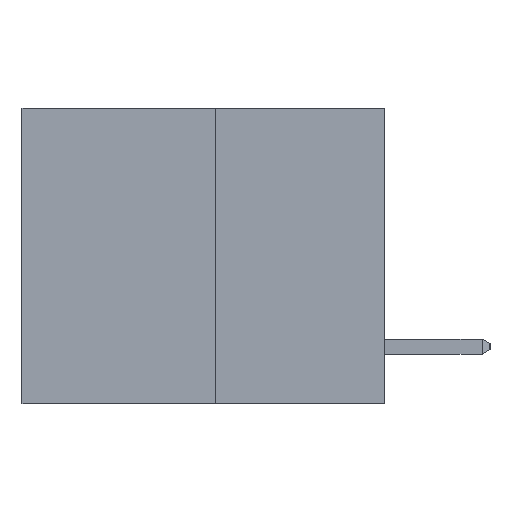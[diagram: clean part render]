
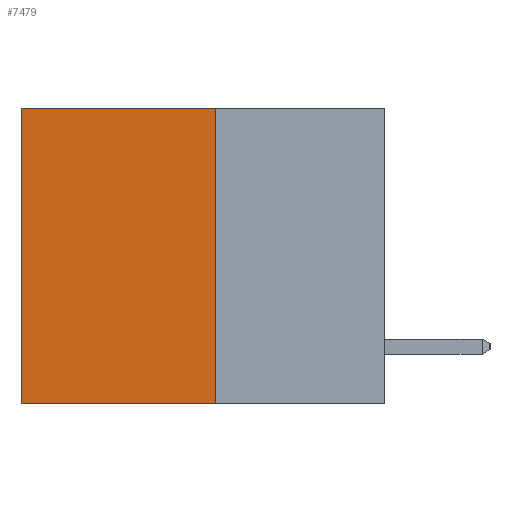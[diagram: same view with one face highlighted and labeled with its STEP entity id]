
A CAD part, left-side view. The second image highlights one B-rep face of the part: STEP entity #7479.
In plain terms, the highlighted planar face has unit normal (-1, 0, 0).
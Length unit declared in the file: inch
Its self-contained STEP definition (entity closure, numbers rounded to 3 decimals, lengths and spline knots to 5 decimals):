
#3 = EDGE_CURVE ( 'NONE', #7090, #13410, #5856, .T. ) ;
#806 = DIRECTION ( 'NONE',  ( 0., 0., -1. ) ) ;
#879 = ORIENTED_EDGE ( 'NONE', *, *, #5650, .T. ) ;
#2530 = CARTESIAN_POINT ( 'NONE',  ( 0.3165, 0.28, 0. ) ) ;
#3694 = LINE ( 'NONE', #10502, #8239 ) ;
#3913 = DIRECTION ( 'NONE',  ( 0., 0., -1. ) ) ;
#5212 = CARTESIAN_POINT ( 'NONE',  ( 0.3165, 0.6, -0.49 ) ) ;
#5503 = LINE ( 'NONE', #7113, #12118 ) ;
#5650 = EDGE_CURVE ( 'NONE', #7469, #7090, #3694, .T. ) ;
#5856 = LINE ( 'NONE', #9964, #11544 ) ;
#5932 = EDGE_LOOP ( 'NONE', ( #9068, #12618, #8755, #879 ) ) ;
#6131 = DIRECTION ( 'NONE',  ( 1., 0., 0. ) ) ;
#7090 = VERTEX_POINT ( 'NONE', #12111 ) ;
#7113 = CARTESIAN_POINT ( 'NONE',  ( 0.3165, 0.28, -0.49 ) ) ;
#7469 = VERTEX_POINT ( 'NONE', #2530 ) ;
#7479 = ADVANCED_FACE ( 'NONE', ( #7515 ), #10702, .F. ) ;
#7515 = FACE_OUTER_BOUND ( 'NONE', #5932, .T. ) ;
#7644 = EDGE_CURVE ( 'NONE', #7469, #12698, #12450, .T. ) ;
#8082 = DIRECTION ( 'NONE',  ( 0., 1., 0. ) ) ;
#8239 = VECTOR ( 'NONE', #8082, 39.37008 ) ;
#8270 = DIRECTION ( 'NONE',  ( 0., 1., 0. ) ) ;
#8755 = ORIENTED_EDGE ( 'NONE', *, *, #7644, .F. ) ;
#8775 = DIRECTION ( 'NONE',  ( 0., 0., -1. ) ) ;
#9068 = ORIENTED_EDGE ( 'NONE', *, *, #3, .T. ) ;
#9707 = AXIS2_PLACEMENT_3D ( 'NONE', #10960, #6131, #3913 ) ;
#9881 = VECTOR ( 'NONE', #8775, 39.37008 ) ;
#9964 = CARTESIAN_POINT ( 'NONE',  ( 0.3165, 0.6, -0.49 ) ) ;
#10502 = CARTESIAN_POINT ( 'NONE',  ( 0.3165, 0.28, 0. ) ) ;
#10702 = PLANE ( 'NONE',  #9707 ) ;
#10960 = CARTESIAN_POINT ( 'NONE',  ( 0.3165, 0.28, -0.49 ) ) ;
#11544 = VECTOR ( 'NONE', #806, 39.37008 ) ;
#12111 = CARTESIAN_POINT ( 'NONE',  ( 0.3165, 0.6, 0. ) ) ;
#12118 = VECTOR ( 'NONE', #8270, 39.37008 ) ;
#12277 = CARTESIAN_POINT ( 'NONE',  ( 0.3165, 0.28, -0.49 ) ) ;
#12450 = LINE ( 'NONE', #12277, #9881 ) ;
#12618 = ORIENTED_EDGE ( 'NONE', *, *, #13878, .F. ) ;
#12698 = VERTEX_POINT ( 'NONE', #14039 ) ;
#13410 = VERTEX_POINT ( 'NONE', #5212 ) ;
#13878 = EDGE_CURVE ( 'NONE', #12698, #13410, #5503, .T. ) ;
#14039 = CARTESIAN_POINT ( 'NONE',  ( 0.3165, 0.28, -0.49 ) ) ;
